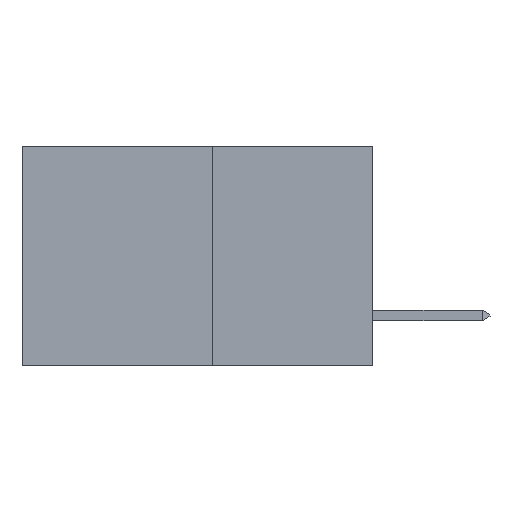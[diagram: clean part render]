
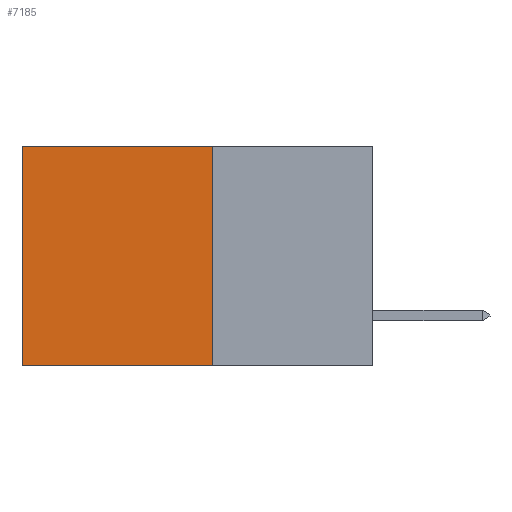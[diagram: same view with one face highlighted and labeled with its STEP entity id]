
A CAD part, left-side view. The second image highlights one B-rep face of the part: STEP entity #7185.
In plain terms, the highlighted planar face has unit normal (-1, 0, 0).
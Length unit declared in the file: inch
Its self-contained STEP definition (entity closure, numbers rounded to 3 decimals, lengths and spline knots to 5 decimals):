
#2 = CARTESIAN_POINT ( 'NONE',  ( 0.277, 0.27, -0.37 ) ) ;
#66 = DIRECTION ( 'NONE',  ( 0., 1., 0. ) ) ;
#306 = ORIENTED_EDGE ( 'NONE', *, *, #5024, .T. ) ;
#1727 = AXIS2_PLACEMENT_3D ( 'NONE', #7454, #7355, #7320 ) ;
#1760 = ORIENTED_EDGE ( 'NONE', *, *, #3262, .F. ) ;
#2283 = ORIENTED_EDGE ( 'NONE', *, *, #6955, .F. ) ;
#2516 = CARTESIAN_POINT ( 'NONE',  ( 0.277, 0.59, 0. ) ) ;
#2624 = LINE ( 'NONE', #3099, #9088 ) ;
#2683 = ORIENTED_EDGE ( 'NONE', *, *, #7864, .T. ) ;
#2780 = VERTEX_POINT ( 'NONE', #4550 ) ;
#2807 = EDGE_LOOP ( 'NONE', ( #2683, #2283, #1760, #306 ) ) ;
#3099 = CARTESIAN_POINT ( 'NONE',  ( 0.277, 0.27, -0.37 ) ) ;
#3152 = LINE ( 'NONE', #10139, #9840 ) ;
#3177 = DIRECTION ( 'NONE',  ( 0., 0., -1. ) ) ;
#3262 = EDGE_CURVE ( 'NONE', #3834, #9293, #2624, .T. ) ;
#3834 = VERTEX_POINT ( 'NONE', #10094 ) ;
#4318 = CARTESIAN_POINT ( 'NONE',  ( 0.277, 0.27, -0.37 ) ) ;
#4349 = LINE ( 'NONE', #2, #10669 ) ;
#4550 = CARTESIAN_POINT ( 'NONE',  ( 0.277, 0.59, -0.37 ) ) ;
#5024 = EDGE_CURVE ( 'NONE', #3834, #5335, #3152, .T. ) ;
#5161 = DIRECTION ( 'NONE',  ( 0., 0., -1. ) ) ;
#5335 = VERTEX_POINT ( 'NONE', #2516 ) ;
#6121 = LINE ( 'NONE', #10825, #10648 ) ;
#6955 = EDGE_CURVE ( 'NONE', #9293, #2780, #4349, .T. ) ;
#7185 = ADVANCED_FACE ( 'NONE', ( #8643 ), #8072, .F. ) ;
#7320 = DIRECTION ( 'NONE',  ( 0., 0., -1. ) ) ;
#7355 = DIRECTION ( 'NONE',  ( 1., 0., 0. ) ) ;
#7454 = CARTESIAN_POINT ( 'NONE',  ( 0.277, 0.27, -0.37 ) ) ;
#7864 = EDGE_CURVE ( 'NONE', #5335, #2780, #6121, .T. ) ;
#8072 = PLANE ( 'NONE',  #1727 ) ;
#8643 = FACE_OUTER_BOUND ( 'NONE', #2807, .T. ) ;
#9088 = VECTOR ( 'NONE', #3177, 39.37008 ) ;
#9293 = VERTEX_POINT ( 'NONE', #4318 ) ;
#9733 = DIRECTION ( 'NONE',  ( 0., 1., 0. ) ) ;
#9840 = VECTOR ( 'NONE', #9733, 39.37008 ) ;
#10094 = CARTESIAN_POINT ( 'NONE',  ( 0.277, 0.27, 0. ) ) ;
#10139 = CARTESIAN_POINT ( 'NONE',  ( 0.277, 0.27, 0. ) ) ;
#10648 = VECTOR ( 'NONE', #5161, 39.37008 ) ;
#10669 = VECTOR ( 'NONE', #66, 39.37008 ) ;
#10825 = CARTESIAN_POINT ( 'NONE',  ( 0.277, 0.59, -0.37 ) ) ;
